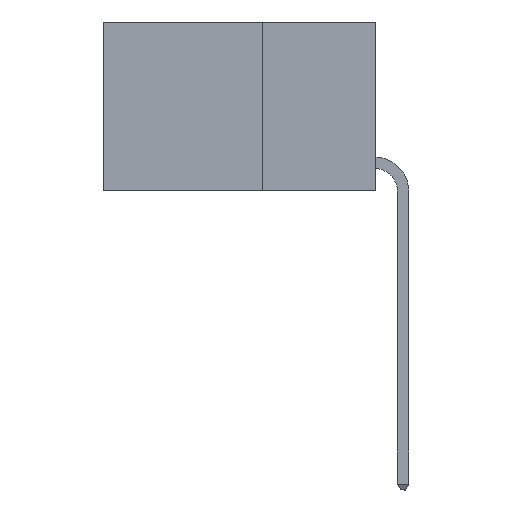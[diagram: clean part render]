
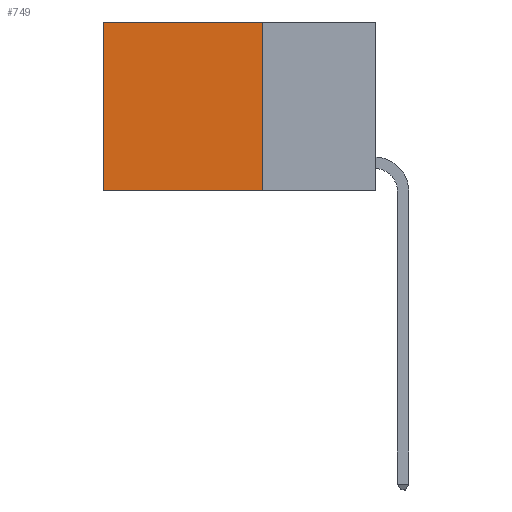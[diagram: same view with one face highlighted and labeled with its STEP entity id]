
A CAD part, left-side view. The second image highlights one B-rep face of the part: STEP entity #749.
In plain terms, the highlighted planar face has unit normal (-1, 0, 0).
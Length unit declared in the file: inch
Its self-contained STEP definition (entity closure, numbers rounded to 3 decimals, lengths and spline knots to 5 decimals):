
#131 = ORIENTED_EDGE ( 'NONE', *, *, #6977, .T. ) ;
#445 = EDGE_CURVE ( 'NONE', #11059, #6101, #15604, .T. ) ;
#749 = ADVANCED_FACE ( 'NONE', ( #11612 ), #5335, .F. ) ;
#1052 = LINE ( 'NONE', #1542, #3932 ) ;
#1480 = DIRECTION ( 'NONE',  ( 0., 0., -1. ) ) ;
#1542 = CARTESIAN_POINT ( 'NONE',  ( 0.2625, 0.25, 0. ) ) ;
#1568 = EDGE_CURVE ( 'NONE', #8408, #11059, #1052, .T. ) ;
#2000 = EDGE_LOOP ( 'NONE', ( #131, #9844, #4408, #10620 ) ) ;
#2501 = LINE ( 'NONE', #5781, #5639 ) ;
#2717 = DIRECTION ( 'NONE',  ( 0., 0., -1. ) ) ;
#2903 = DIRECTION ( 'NONE',  ( 0., 1., 0. ) ) ;
#3932 = VECTOR ( 'NONE', #1480, 39.37008 ) ;
#4408 = ORIENTED_EDGE ( 'NONE', *, *, #1568, .F. ) ;
#5335 = PLANE ( 'NONE',  #12483 ) ;
#5451 = VECTOR ( 'NONE', #2903, 39.37008 ) ;
#5639 = VECTOR ( 'NONE', #12406, 39.37008 ) ;
#5781 = CARTESIAN_POINT ( 'NONE',  ( 0.2625, 0.6, 0. ) ) ;
#5840 = LINE ( 'NONE', #15921, #5451 ) ;
#6017 = CARTESIAN_POINT ( 'NONE',  ( 0.2625, 0.6, -0.37 ) ) ;
#6101 = VERTEX_POINT ( 'NONE', #6017 ) ;
#6955 = VERTEX_POINT ( 'NONE', #16152 ) ;
#6977 = EDGE_CURVE ( 'NONE', #6955, #6101, #2501, .T. ) ;
#8408 = VERTEX_POINT ( 'NONE', #14118 ) ;
#9844 = ORIENTED_EDGE ( 'NONE', *, *, #445, .F. ) ;
#10620 = ORIENTED_EDGE ( 'NONE', *, *, #11909, .T. ) ;
#10656 = DIRECTION ( 'NONE',  ( 1., 0., 0. ) ) ;
#11059 = VERTEX_POINT ( 'NONE', #14165 ) ;
#11362 = CARTESIAN_POINT ( 'NONE',  ( 0.2625, 0.25, -0.37 ) ) ;
#11612 = FACE_OUTER_BOUND ( 'NONE', #2000, .T. ) ;
#11909 = EDGE_CURVE ( 'NONE', #8408, #6955, #5840, .T. ) ;
#12406 = DIRECTION ( 'NONE',  ( 0., 0., -1. ) ) ;
#12483 = AXIS2_PLACEMENT_3D ( 'NONE', #14512, #10656, #2717 ) ;
#12692 = DIRECTION ( 'NONE',  ( 0., 1., 0. ) ) ;
#14118 = CARTESIAN_POINT ( 'NONE',  ( 0.2625, 0.25, 0. ) ) ;
#14165 = CARTESIAN_POINT ( 'NONE',  ( 0.2625, 0.25, -0.37 ) ) ;
#14512 = CARTESIAN_POINT ( 'NONE',  ( 0.2625, 0.25, 0. ) ) ;
#15203 = VECTOR ( 'NONE', #12692, 39.37008 ) ;
#15604 = LINE ( 'NONE', #11362, #15203 ) ;
#15921 = CARTESIAN_POINT ( 'NONE',  ( 0.2625, 0.25, 0. ) ) ;
#16152 = CARTESIAN_POINT ( 'NONE',  ( 0.2625, 0.6, 0. ) ) ;
